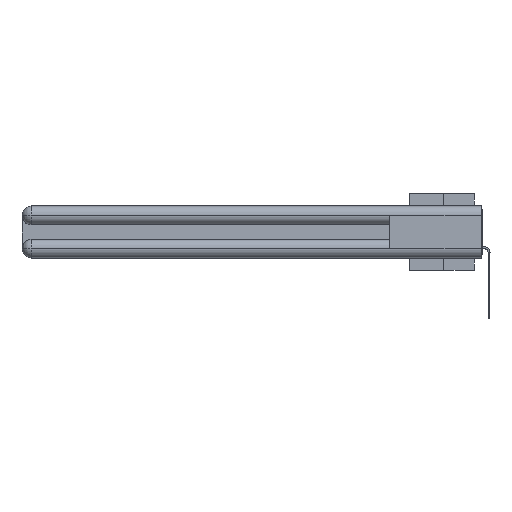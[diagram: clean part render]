
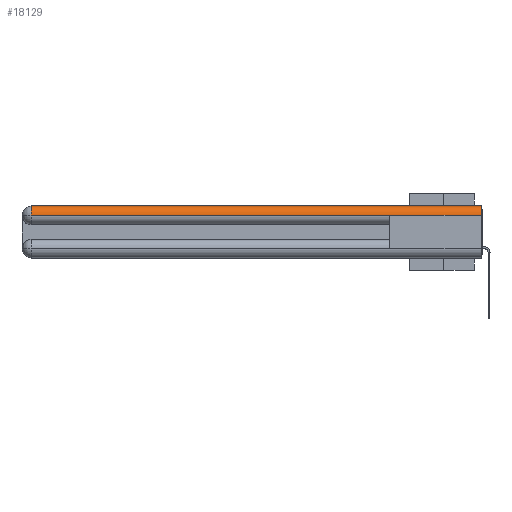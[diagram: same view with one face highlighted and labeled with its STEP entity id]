
A CAD part, left-side view. The second image highlights one B-rep face of the part: STEP entity #18129.
In plain terms, the highlighted cylindrical face has radius 1.562 mm (diameter 3.124 mm), a partial arc.
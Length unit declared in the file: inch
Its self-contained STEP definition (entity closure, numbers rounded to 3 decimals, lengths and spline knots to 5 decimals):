
#85 = AXIS2_PLACEMENT_3D ( 'NONE', #3934, #13187, #4232 ) ;
#1643 = CARTESIAN_POINT ( 'NONE',  ( 0., 2.94, -0.0615 ) ) ;
#2023 = LINE ( 'NONE', #25086, #2671 ) ;
#2138 = VECTOR ( 'NONE', #18229, 39.37008 ) ;
#2591 = LINE ( 'NONE', #9574, #20236 ) ;
#2595 = ORIENTED_EDGE ( 'NONE', *, *, #9344, .F. ) ;
#2671 = VECTOR ( 'NONE', #13541, 39.37008 ) ;
#3124 = CIRCLE ( 'NONE', #4552, 0.0615 ) ;
#3144 = EDGE_CURVE ( 'NONE', #27544, #12021, #2591, .T. ) ;
#3934 = CARTESIAN_POINT ( 'NONE',  ( 0.0615, 2.94, -0.0615 ) ) ;
#4183 = ORIENTED_EDGE ( 'NONE', *, *, #22314, .F. ) ;
#4232 = DIRECTION ( 'NONE',  ( 0., 0., 1. ) ) ;
#4552 = AXIS2_PLACEMENT_3D ( 'NONE', #22639, #13816, #11554 ) ;
#6313 = ORIENTED_EDGE ( 'NONE', *, *, #22315, .F. ) ;
#7148 = VERTEX_POINT ( 'NONE', #11613 ) ;
#9344 = EDGE_CURVE ( 'NONE', #7148, #12011, #2023, .T. ) ;
#9574 = CARTESIAN_POINT ( 'NONE',  ( 0., 3., -0.0615 ) ) ;
#9759 = CIRCLE ( 'NONE', #85, 0.0615 ) ;
#10463 = DIRECTION ( 'NONE',  ( 0., 0., 1. ) ) ;
#11554 = DIRECTION ( 'NONE',  ( 1., 0., 0. ) ) ;
#11613 = CARTESIAN_POINT ( 'NONE',  ( 0.0615, 2.94, 0. ) ) ;
#12011 = VERTEX_POINT ( 'NONE', #16191 ) ;
#12021 = VERTEX_POINT ( 'NONE', #12087 ) ;
#12087 = CARTESIAN_POINT ( 'NONE',  ( 0., 0.6, -0.0615 ) ) ;
#13187 = DIRECTION ( 'NONE',  ( 0., -1., 0. ) ) ;
#13541 = DIRECTION ( 'NONE',  ( 0., -1., 0. ) ) ;
#13659 = EDGE_LOOP ( 'NONE', ( #2595, #14493, #28119, #6313, #4183 ) ) ;
#13816 = DIRECTION ( 'NONE',  ( 0., -1., 0. ) ) ;
#14493 = ORIENTED_EDGE ( 'NONE', *, *, #17837, .T. ) ;
#16191 = CARTESIAN_POINT ( 'NONE',  ( 0.0615, 0., 0. ) ) ;
#17837 = EDGE_CURVE ( 'NONE', #7148, #27544, #9759, .T. ) ;
#18129 = ADVANCED_FACE ( 'NONE', ( #26668 ), #28513, .T. ) ;
#18229 = DIRECTION ( 'NONE',  ( 0., 1., 0. ) ) ;
#19438 = AXIS2_PLACEMENT_3D ( 'NONE', #23804, #26523, #10463 ) ;
#20236 = VECTOR ( 'NONE', #20801, 39.37008 ) ;
#20352 = LINE ( 'NONE', #27330, #2138 ) ;
#20801 = DIRECTION ( 'NONE',  ( 0., -1., 0. ) ) ;
#22314 = EDGE_CURVE ( 'NONE', #12011, #24229, #3124, .T. ) ;
#22315 = EDGE_CURVE ( 'NONE', #24229, #12021, #20352, .T. ) ;
#22639 = CARTESIAN_POINT ( 'NONE',  ( 0.0615, 0., -0.0615 ) ) ;
#23804 = CARTESIAN_POINT ( 'NONE',  ( 0.0615, 0., -0.0615 ) ) ;
#24229 = VERTEX_POINT ( 'NONE', #29527 ) ;
#25086 = CARTESIAN_POINT ( 'NONE',  ( 0.0615, 0., 0. ) ) ;
#26523 = DIRECTION ( 'NONE',  ( 0., 1., 0. ) ) ;
#26668 = FACE_OUTER_BOUND ( 'NONE', #13659, .T. ) ;
#27330 = CARTESIAN_POINT ( 'NONE',  ( 0., 3., -0.0615 ) ) ;
#27544 = VERTEX_POINT ( 'NONE', #1643 ) ;
#28119 = ORIENTED_EDGE ( 'NONE', *, *, #3144, .T. ) ;
#28513 = CYLINDRICAL_SURFACE ( 'NONE', #19438, 0.0615 ) ;
#29527 = CARTESIAN_POINT ( 'NONE',  ( 0., 0., -0.0615 ) ) ;
